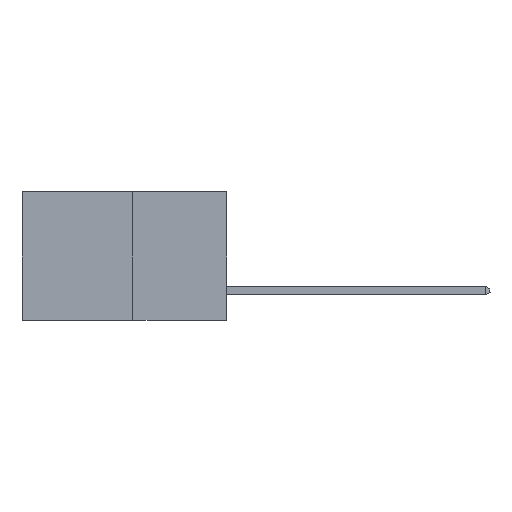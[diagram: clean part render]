
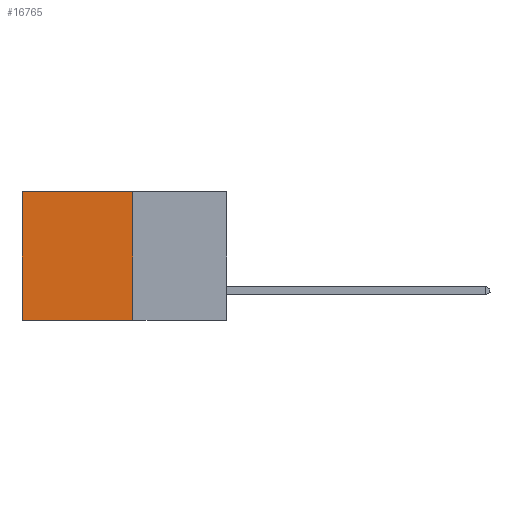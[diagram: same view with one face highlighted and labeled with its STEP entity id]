
A CAD part, left-side view. The second image highlights one B-rep face of the part: STEP entity #16765.
In plain terms, the highlighted planar face has unit normal (-1, 0, 0).
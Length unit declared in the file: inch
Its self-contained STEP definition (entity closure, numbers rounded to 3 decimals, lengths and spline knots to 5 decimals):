
#608 = ORIENTED_EDGE ( 'NONE', *, *, #5738, .T. ) ;
#2105 = FACE_OUTER_BOUND ( 'NONE', #3170, .T. ) ;
#2253 = VERTEX_POINT ( 'NONE', #17416 ) ;
#3170 = EDGE_LOOP ( 'NONE', ( #608, #17083, #5923, #13923 ) ) ;
#3969 = DIRECTION ( 'NONE',  ( 0., 0., -1. ) ) ;
#4778 = CARTESIAN_POINT ( 'NONE',  ( 0.277, 0.59, -0.37 ) ) ;
#4936 = DIRECTION ( 'NONE',  ( 1., 0., 0. ) ) ;
#4982 = LINE ( 'NONE', #18475, #17306 ) ;
#5738 = EDGE_CURVE ( 'NONE', #2253, #16382, #18130, .T. ) ;
#5793 = CARTESIAN_POINT ( 'NONE',  ( 0.277, 0.59, -0.37 ) ) ;
#5923 = ORIENTED_EDGE ( 'NONE', *, *, #19445, .F. ) ;
#6049 = VECTOR ( 'NONE', #3969, 39.37008 ) ;
#7322 = CARTESIAN_POINT ( 'NONE',  ( 0.277, 0.27, 0. ) ) ;
#8410 = CARTESIAN_POINT ( 'NONE',  ( 0.277, 0.27, -0.37 ) ) ;
#8435 = DIRECTION ( 'NONE',  ( 0., 1., 0. ) ) ;
#9097 = VECTOR ( 'NONE', #8435, 39.37008 ) ;
#9386 = AXIS2_PLACEMENT_3D ( 'NONE', #8410, #4936, #11812 ) ;
#9936 = EDGE_CURVE ( 'NONE', #13098, #2253, #18119, .T. ) ;
#10098 = DIRECTION ( 'NONE',  ( 0., 0., -1. ) ) ;
#10126 = PLANE ( 'NONE',  #9386 ) ;
#11202 = EDGE_CURVE ( 'NONE', #12759, #16382, #4982, .T. ) ;
#11565 = CARTESIAN_POINT ( 'NONE',  ( 0.277, 0.27, -0.37 ) ) ;
#11812 = DIRECTION ( 'NONE',  ( 0., 0., -1. ) ) ;
#12759 = VERTEX_POINT ( 'NONE', #11565 ) ;
#13098 = VERTEX_POINT ( 'NONE', #7322 ) ;
#13400 = DIRECTION ( 'NONE',  ( 0., 1., 0. ) ) ;
#13451 = CARTESIAN_POINT ( 'NONE',  ( 0.277, 0.27, 0. ) ) ;
#13587 = VECTOR ( 'NONE', #10098, 39.37008 ) ;
#13923 = ORIENTED_EDGE ( 'NONE', *, *, #9936, .T. ) ;
#16382 = VERTEX_POINT ( 'NONE', #5793 ) ;
#16765 = ADVANCED_FACE ( 'NONE', ( #2105 ), #10126, .F. ) ;
#17083 = ORIENTED_EDGE ( 'NONE', *, *, #11202, .F. ) ;
#17306 = VECTOR ( 'NONE', #13400, 39.37008 ) ;
#17416 = CARTESIAN_POINT ( 'NONE',  ( 0.277, 0.59, 0. ) ) ;
#18119 = LINE ( 'NONE', #13451, #9097 ) ;
#18130 = LINE ( 'NONE', #4778, #13587 ) ;
#18475 = CARTESIAN_POINT ( 'NONE',  ( 0.277, 0.27, -0.37 ) ) ;
#19445 = EDGE_CURVE ( 'NONE', #13098, #12759, #19606, .T. ) ;
#19606 = LINE ( 'NONE', #20929, #6049 ) ;
#20929 = CARTESIAN_POINT ( 'NONE',  ( 0.277, 0.27, -0.37 ) ) ;
